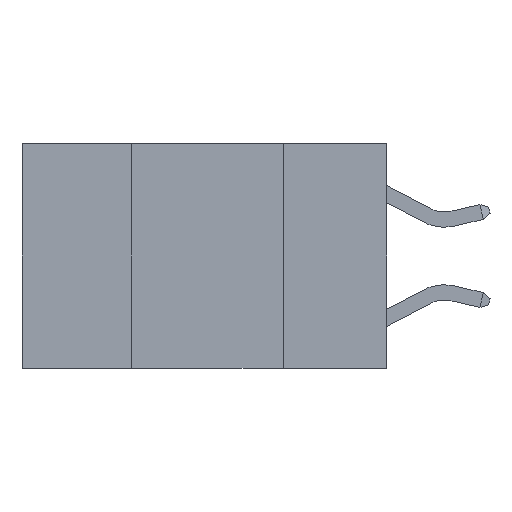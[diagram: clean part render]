
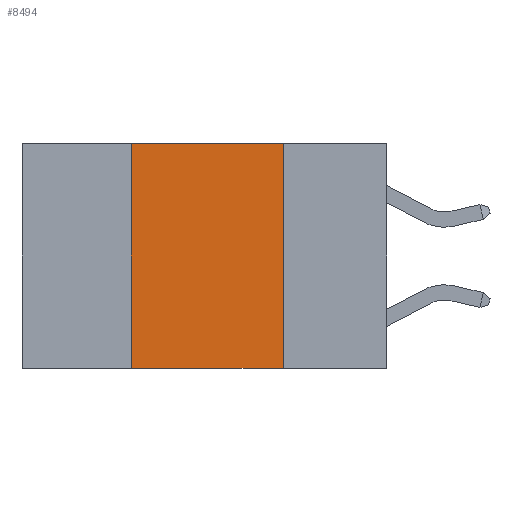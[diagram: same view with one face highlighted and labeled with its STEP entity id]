
A CAD part, left-side view. The second image highlights one B-rep face of the part: STEP entity #8494.
In plain terms, the highlighted planar face has unit normal (-1, 0, 0).
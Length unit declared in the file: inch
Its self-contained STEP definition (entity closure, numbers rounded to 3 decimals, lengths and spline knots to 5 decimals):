
#241 = DIRECTION ( 'NONE',  ( 0., -1., 0. ) ) ;
#569 = VERTEX_POINT ( 'NONE', #1755 ) ;
#1050 = VECTOR ( 'NONE', #5496, 39.37008 ) ;
#1538 = VERTEX_POINT ( 'NONE', #9841 ) ;
#1755 = CARTESIAN_POINT ( 'NONE',  ( 0., 0.42, 0. ) ) ;
#1829 = VECTOR ( 'NONE', #10726, 39.37008 ) ;
#2071 = EDGE_CURVE ( 'NONE', #1538, #569, #13454, .T. ) ;
#2467 = DIRECTION ( 'NONE',  ( 0., 0., -1. ) ) ;
#2679 = EDGE_CURVE ( 'NONE', #1538, #13142, #10018, .T. ) ;
#2833 = EDGE_CURVE ( 'NONE', #569, #7399, #3522, .T. ) ;
#2895 = ORIENTED_EDGE ( 'NONE', *, *, #5209, .F. ) ;
#3381 = CARTESIAN_POINT ( 'NONE',  ( 0., 0.6, -0.37 ) ) ;
#3522 = LINE ( 'NONE', #8105, #8859 ) ;
#3705 = EDGE_LOOP ( 'NONE', ( #2895, #5198, #5754, #6068 ) ) ;
#5198 = ORIENTED_EDGE ( 'NONE', *, *, #2833, .F. ) ;
#5209 = EDGE_CURVE ( 'NONE', #7399, #13142, #10950, .T. ) ;
#5280 = CARTESIAN_POINT ( 'NONE',  ( 0., 0.17, 0. ) ) ;
#5496 = DIRECTION ( 'NONE',  ( 0., 0., 1. ) ) ;
#5754 = ORIENTED_EDGE ( 'NONE', *, *, #2071, .F. ) ;
#5843 = DIRECTION ( 'NONE',  ( 1., 0., 0. ) ) ;
#6068 = ORIENTED_EDGE ( 'NONE', *, *, #2679, .T. ) ;
#6137 = AXIS2_PLACEMENT_3D ( 'NONE', #13501, #5843, #2467 ) ;
#7301 = CARTESIAN_POINT ( 'NONE',  ( 0., 0.17, 0. ) ) ;
#7399 = VERTEX_POINT ( 'NONE', #7301 ) ;
#8105 = CARTESIAN_POINT ( 'NONE',  ( 0., 0.6, 0. ) ) ;
#8494 = ADVANCED_FACE ( 'NONE', ( #11423 ), #10153, .F. ) ;
#8777 = CARTESIAN_POINT ( 'NONE',  ( 0., 0.42, 0. ) ) ;
#8859 = VECTOR ( 'NONE', #241, 39.37008 ) ;
#9841 = CARTESIAN_POINT ( 'NONE',  ( 0., 0.42, -0.37 ) ) ;
#10018 = LINE ( 'NONE', #3381, #13350 ) ;
#10153 = PLANE ( 'NONE',  #6137 ) ;
#10726 = DIRECTION ( 'NONE',  ( 0., 0., -1. ) ) ;
#10950 = LINE ( 'NONE', #5280, #1829 ) ;
#11423 = FACE_OUTER_BOUND ( 'NONE', #3705, .T. ) ;
#12316 = DIRECTION ( 'NONE',  ( 0., -1., 0. ) ) ;
#13142 = VERTEX_POINT ( 'NONE', #14380 ) ;
#13350 = VECTOR ( 'NONE', #12316, 39.37008 ) ;
#13454 = LINE ( 'NONE', #8777, #1050 ) ;
#13501 = CARTESIAN_POINT ( 'NONE',  ( 0., 0.6, 0. ) ) ;
#14380 = CARTESIAN_POINT ( 'NONE',  ( 0., 0.17, -0.37 ) ) ;
